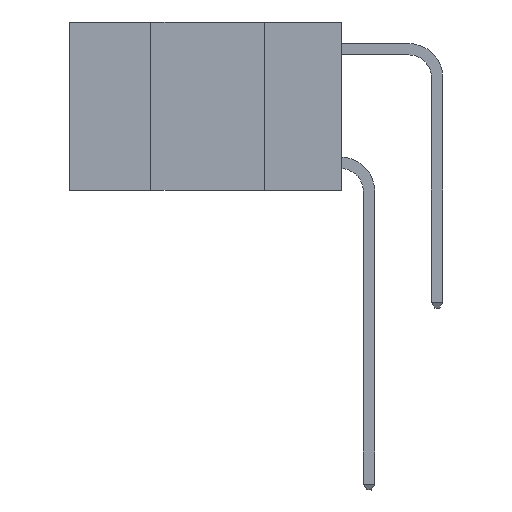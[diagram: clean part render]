
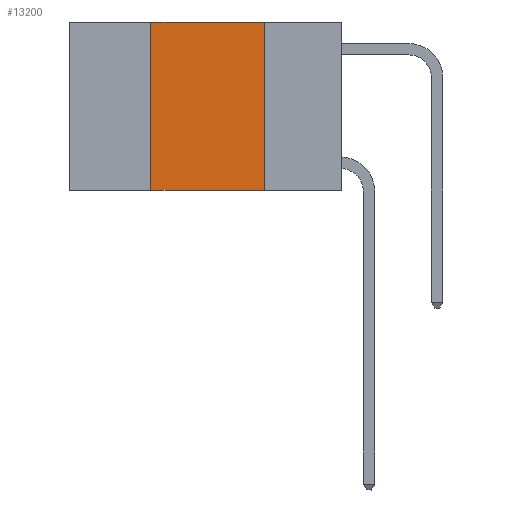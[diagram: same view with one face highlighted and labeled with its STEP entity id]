
A CAD part, left-side view. The second image highlights one B-rep face of the part: STEP entity #13200.
In plain terms, the highlighted planar face has unit normal (-1, 0, 0).
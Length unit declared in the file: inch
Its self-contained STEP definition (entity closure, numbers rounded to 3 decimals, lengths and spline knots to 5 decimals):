
#586 = CARTESIAN_POINT ( 'NONE',  ( 0., 0.6, 0. ) ) ;
#678 = VECTOR ( 'NONE', #18658, 39.37008 ) ;
#982 = VECTOR ( 'NONE', #20081, 39.37008 ) ;
#1069 = LINE ( 'NONE', #15705, #14078 ) ;
#1281 = ORIENTED_EDGE ( 'NONE', *, *, #3657, .F. ) ;
#2714 = VERTEX_POINT ( 'NONE', #2961 ) ;
#2961 = CARTESIAN_POINT ( 'NONE',  ( 0., 0.17, -0.37 ) ) ;
#3639 = CARTESIAN_POINT ( 'NONE',  ( 0., 0.42, 0. ) ) ;
#3657 = EDGE_CURVE ( 'NONE', #11532, #14261, #19070, .T. ) ;
#3754 = DIRECTION ( 'NONE',  ( 0., 0., 1. ) ) ;
#4001 = DIRECTION ( 'NONE',  ( 0., 0., -1. ) ) ;
#4756 = EDGE_LOOP ( 'NONE', ( #9750, #1281, #14833, #6331 ) ) ;
#5015 = AXIS2_PLACEMENT_3D ( 'NONE', #586, #14159, #4001 ) ;
#5158 = LINE ( 'NONE', #16907, #678 ) ;
#5615 = PLANE ( 'NONE',  #5015 ) ;
#6331 = ORIENTED_EDGE ( 'NONE', *, *, #21570, .T. ) ;
#7804 = FACE_OUTER_BOUND ( 'NONE', #4756, .T. ) ;
#9750 = ORIENTED_EDGE ( 'NONE', *, *, #19184, .F. ) ;
#10281 = VERTEX_POINT ( 'NONE', #10845 ) ;
#10845 = CARTESIAN_POINT ( 'NONE',  ( 0., 0.42, -0.37 ) ) ;
#11532 = VERTEX_POINT ( 'NONE', #3639 ) ;
#11774 = LINE ( 'NONE', #13587, #20917 ) ;
#13200 = ADVANCED_FACE ( 'NONE', ( #7804 ), #5615, .F. ) ;
#13587 = CARTESIAN_POINT ( 'NONE',  ( 0., 0.42, 0. ) ) ;
#14078 = VECTOR ( 'NONE', #15783, 39.37008 ) ;
#14159 = DIRECTION ( 'NONE',  ( 1., 0., 0. ) ) ;
#14261 = VERTEX_POINT ( 'NONE', #21907 ) ;
#14833 = ORIENTED_EDGE ( 'NONE', *, *, #20387, .F. ) ;
#15705 = CARTESIAN_POINT ( 'NONE',  ( 0., 0.6, -0.37 ) ) ;
#15783 = DIRECTION ( 'NONE',  ( 0., -1., 0. ) ) ;
#16907 = CARTESIAN_POINT ( 'NONE',  ( 0., 0.17, 0. ) ) ;
#17499 = CARTESIAN_POINT ( 'NONE',  ( 0., 0.6, 0. ) ) ;
#18658 = DIRECTION ( 'NONE',  ( 0., 0., -1. ) ) ;
#19070 = LINE ( 'NONE', #17499, #982 ) ;
#19184 = EDGE_CURVE ( 'NONE', #14261, #2714, #5158, .T. ) ;
#20081 = DIRECTION ( 'NONE',  ( 0., -1., 0. ) ) ;
#20387 = EDGE_CURVE ( 'NONE', #10281, #11532, #11774, .T. ) ;
#20917 = VECTOR ( 'NONE', #3754, 39.37008 ) ;
#21570 = EDGE_CURVE ( 'NONE', #10281, #2714, #1069, .T. ) ;
#21907 = CARTESIAN_POINT ( 'NONE',  ( 0., 0.17, 0. ) ) ;
